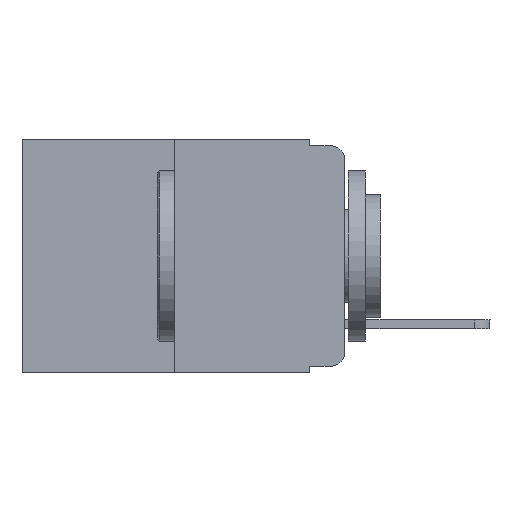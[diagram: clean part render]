
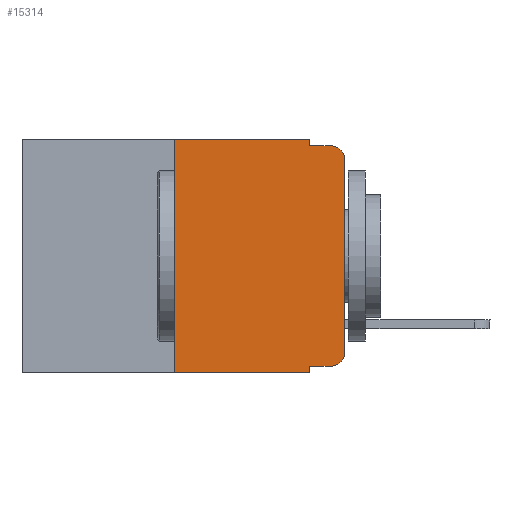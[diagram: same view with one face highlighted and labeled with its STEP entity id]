
A CAD part, left-side view. The second image highlights one B-rep face of the part: STEP entity #15314.
In plain terms, the highlighted planar face has unit normal (-1, 0, 0).
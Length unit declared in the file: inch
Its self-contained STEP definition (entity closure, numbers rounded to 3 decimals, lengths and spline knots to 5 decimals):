
#83 = CARTESIAN_POINT ( 'NONE',  ( 0., 0.25, 0. ) ) ;
#337 = VERTEX_POINT ( 'NONE', #5318 ) ;
#509 = DIRECTION ( 'NONE',  ( 0., -1., 0. ) ) ;
#611 = VECTOR ( 'NONE', #786, 39.37008 ) ;
#786 = DIRECTION ( 'NONE',  ( 0., -1., 0. ) ) ;
#1023 = CARTESIAN_POINT ( 'NONE',  ( 0., 0.02, -0.333 ) ) ;
#1964 = DIRECTION ( 'NONE',  ( 0., 0., 1. ) ) ;
#2170 = LINE ( 'NONE', #18024, #13381 ) ;
#2611 = CARTESIAN_POINT ( 'NONE',  ( 0., 0.25, 0. ) ) ;
#2786 = EDGE_CURVE ( 'NONE', #10088, #16052, #11819, .T. ) ;
#2987 = VECTOR ( 'NONE', #15425, 39.37008 ) ;
#3305 = VERTEX_POINT ( 'NONE', #14002 ) ;
#3441 = CARTESIAN_POINT ( 'NONE',  ( 0., 0.051, 0. ) ) ;
#3513 = CARTESIAN_POINT ( 'NONE',  ( 0., 0.02, -0.03 ) ) ;
#3536 = LINE ( 'NONE', #8702, #19836 ) ;
#3833 = DIRECTION ( 'NONE',  ( -1., 0., 0. ) ) ;
#4612 = CARTESIAN_POINT ( 'NONE',  ( 0., 0.02, -0.313 ) ) ;
#4723 = ORIENTED_EDGE ( 'NONE', *, *, #2786, .F. ) ;
#4869 = LINE ( 'NONE', #11123, #4875 ) ;
#4875 = VECTOR ( 'NONE', #17794, 39.37008 ) ;
#5318 = CARTESIAN_POINT ( 'NONE',  ( 0., 0.02, -0.01 ) ) ;
#5512 = PLANE ( 'NONE',  #19628 ) ;
#5529 = CARTESIAN_POINT ( 'NONE',  ( 0., 0.473, 0. ) ) ;
#5636 = LINE ( 'NONE', #5529, #611 ) ;
#5694 = VERTEX_POINT ( 'NONE', #11296 ) ;
#5786 = EDGE_CURVE ( 'NONE', #17242, #5694, #8736, .T. ) ;
#6075 = EDGE_CURVE ( 'NONE', #8983, #9132, #17939, .T. ) ;
#6091 = CIRCLE ( 'NONE', #16245, 0.02 ) ;
#6321 = EDGE_CURVE ( 'NONE', #10088, #5694, #4869, .T. ) ;
#6843 = EDGE_LOOP ( 'NONE', ( #13233, #7590, #18497, #18289, #20855, #4723, #11259, #11020, #12190, #14484 ) ) ;
#6880 = FACE_OUTER_BOUND ( 'NONE', #6843, .T. ) ;
#6923 = VERTEX_POINT ( 'NONE', #9799 ) ;
#6980 = CARTESIAN_POINT ( 'NONE',  ( 0., 0.051, -0.01 ) ) ;
#7224 = CARTESIAN_POINT ( 'NONE',  ( 0., 0.25, -0.343 ) ) ;
#7590 = ORIENTED_EDGE ( 'NONE', *, *, #18512, .T. ) ;
#8702 = CARTESIAN_POINT ( 'NONE',  ( 0., 0.051, -0.01 ) ) ;
#8736 = LINE ( 'NONE', #13732, #12511 ) ;
#8827 = CARTESIAN_POINT ( 'NONE',  ( 0., 0.051, -0.333 ) ) ;
#8983 = VERTEX_POINT ( 'NONE', #16307 ) ;
#9132 = VERTEX_POINT ( 'NONE', #6980 ) ;
#9799 = CARTESIAN_POINT ( 'NONE',  ( 0., 0., -0.313 ) ) ;
#9909 = VECTOR ( 'NONE', #509, 39.37008 ) ;
#10088 = VERTEX_POINT ( 'NONE', #7224 ) ;
#10330 = EDGE_CURVE ( 'NONE', #6923, #3305, #2170, .T. ) ;
#10563 = CIRCLE ( 'NONE', #13282, 0.02 ) ;
#11020 = ORIENTED_EDGE ( 'NONE', *, *, #5786, .F. ) ;
#11123 = CARTESIAN_POINT ( 'NONE',  ( 0., 0.473, -0.343 ) ) ;
#11259 = ORIENTED_EDGE ( 'NONE', *, *, #6321, .T. ) ;
#11296 = CARTESIAN_POINT ( 'NONE',  ( 0., 0.051, -0.343 ) ) ;
#11373 = VERTEX_POINT ( 'NONE', #1023 ) ;
#11420 = CARTESIAN_POINT ( 'NONE',  ( 0., 0.051, -0.333 ) ) ;
#11470 = DIRECTION ( 'NONE',  ( 0., -1., 0. ) ) ;
#11641 = EDGE_CURVE ( 'NONE', #9132, #337, #3536, .T. ) ;
#11774 = CARTESIAN_POINT ( 'NONE',  ( 0., 0.473, 0. ) ) ;
#11819 = LINE ( 'NONE', #2611, #2987 ) ;
#11849 = EDGE_CURVE ( 'NONE', #16052, #8983, #5636, .T. ) ;
#11919 = LINE ( 'NONE', #8827, #9909 ) ;
#12190 = ORIENTED_EDGE ( 'NONE', *, *, #18944, .T. ) ;
#12326 = DIRECTION ( 'NONE',  ( 0., 0., -1. ) ) ;
#12511 = VECTOR ( 'NONE', #13424, 39.37008 ) ;
#13233 = ORIENTED_EDGE ( 'NONE', *, *, #10330, .T. ) ;
#13282 = AXIS2_PLACEMENT_3D ( 'NONE', #3513, #3833, #18007 ) ;
#13381 = VECTOR ( 'NONE', #1964, 39.37008 ) ;
#13424 = DIRECTION ( 'NONE',  ( 0., 0., -1. ) ) ;
#13471 = DIRECTION ( 'NONE',  ( 0., 0., -1. ) ) ;
#13732 = CARTESIAN_POINT ( 'NONE',  ( 0., 0.051, 0. ) ) ;
#14002 = CARTESIAN_POINT ( 'NONE',  ( 0., 0., -0.03 ) ) ;
#14248 = VECTOR ( 'NONE', #19716, 39.37008 ) ;
#14484 = ORIENTED_EDGE ( 'NONE', *, *, #14718, .T. ) ;
#14718 = EDGE_CURVE ( 'NONE', #11373, #6923, #6091, .T. ) ;
#15314 = ADVANCED_FACE ( 'NONE', ( #6880 ), #5512, .F. ) ;
#15425 = DIRECTION ( 'NONE',  ( 0., 0., 1. ) ) ;
#16052 = VERTEX_POINT ( 'NONE', #83 ) ;
#16245 = AXIS2_PLACEMENT_3D ( 'NONE', #4612, #17526, #12326 ) ;
#16307 = CARTESIAN_POINT ( 'NONE',  ( 0., 0.051, 0. ) ) ;
#17242 = VERTEX_POINT ( 'NONE', #11420 ) ;
#17526 = DIRECTION ( 'NONE',  ( -1., 0., 0. ) ) ;
#17794 = DIRECTION ( 'NONE',  ( 0., -1., 0. ) ) ;
#17939 = LINE ( 'NONE', #3441, #14248 ) ;
#18007 = DIRECTION ( 'NONE',  ( 0., 0., -1. ) ) ;
#18024 = CARTESIAN_POINT ( 'NONE',  ( 0., 0., 0. ) ) ;
#18289 = ORIENTED_EDGE ( 'NONE', *, *, #6075, .F. ) ;
#18421 = DIRECTION ( 'NONE',  ( 1., 0., 0. ) ) ;
#18497 = ORIENTED_EDGE ( 'NONE', *, *, #11641, .F. ) ;
#18512 = EDGE_CURVE ( 'NONE', #3305, #337, #10563, .T. ) ;
#18944 = EDGE_CURVE ( 'NONE', #17242, #11373, #11919, .T. ) ;
#19628 = AXIS2_PLACEMENT_3D ( 'NONE', #11774, #18421, #13471 ) ;
#19716 = DIRECTION ( 'NONE',  ( 0., 0., -1. ) ) ;
#19836 = VECTOR ( 'NONE', #11470, 39.37008 ) ;
#20855 = ORIENTED_EDGE ( 'NONE', *, *, #11849, .F. ) ;
